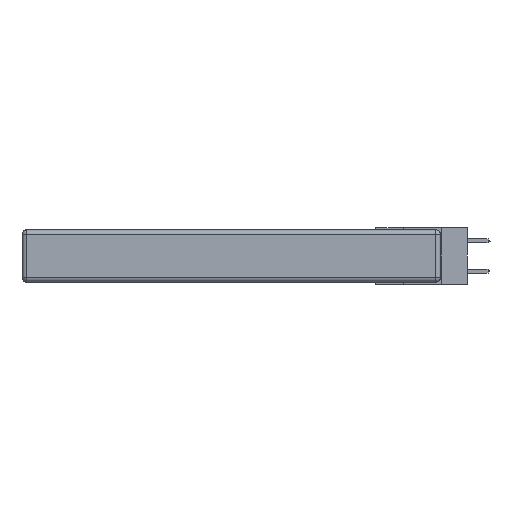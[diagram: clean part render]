
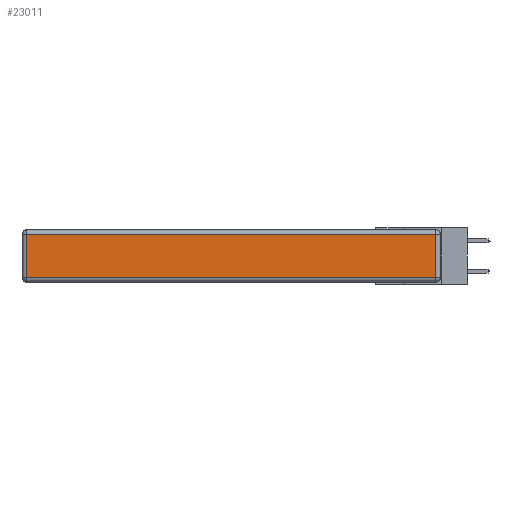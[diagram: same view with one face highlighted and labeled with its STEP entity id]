
A CAD part, left-side view. The second image highlights one B-rep face of the part: STEP entity #23011.
In plain terms, the highlighted planar face has unit normal (-1, 0, 0).
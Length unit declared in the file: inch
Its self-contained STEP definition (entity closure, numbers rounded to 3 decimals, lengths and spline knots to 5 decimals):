
#244 = EDGE_CURVE ( 'NONE', #16506, #13384, #18685, .T. ) ;
#270 = EDGE_CURVE ( 'NONE', #25897, #11508, #22261, .T. ) ;
#1477 = CARTESIAN_POINT ( 'NONE',  ( 0., 2.75, -0.03 ) ) ;
#1549 = ORIENTED_EDGE ( 'NONE', *, *, #270, .T. ) ;
#8575 = DIRECTION ( 'NONE',  ( -1., 0., 0. ) ) ;
#9129 = CARTESIAN_POINT ( 'NONE',  ( 0., 0.03, -0.03 ) ) ;
#9674 = DIRECTION ( 'NONE',  ( 0., 0., -1. ) ) ;
#10591 = VECTOR ( 'NONE', #16017, 39.37008 ) ;
#11338 = DIRECTION ( 'NONE',  ( 0., -1., 0. ) ) ;
#11508 = VERTEX_POINT ( 'NONE', #16377 ) ;
#12030 = ORIENTED_EDGE ( 'NONE', *, *, #14985, .T. ) ;
#13384 = VERTEX_POINT ( 'NONE', #9129 ) ;
#13625 = VECTOR ( 'NONE', #11338, 39.37008 ) ;
#14985 = EDGE_CURVE ( 'NONE', #11508, #16506, #17604, .T. ) ;
#16017 = DIRECTION ( 'NONE',  ( 0., 1., 0. ) ) ;
#16377 = CARTESIAN_POINT ( 'NONE',  ( 0., 2.72, -0.313 ) ) ;
#16506 = VERTEX_POINT ( 'NONE', #28806 ) ;
#16746 = ORIENTED_EDGE ( 'NONE', *, *, #20774, .T. ) ;
#17233 = FACE_OUTER_BOUND ( 'NONE', #24622, .T. ) ;
#17314 = PLANE ( 'NONE',  #20260 ) ;
#17423 = CARTESIAN_POINT ( 'NONE',  ( 0., 0., -0.343 ) ) ;
#17604 = LINE ( 'NONE', #25397, #13625 ) ;
#18685 = LINE ( 'NONE', #23398, #20120 ) ;
#19004 = DIRECTION ( 'NONE',  ( 0., 0., 1. ) ) ;
#19221 = LINE ( 'NONE', #1477, #10591 ) ;
#20120 = VECTOR ( 'NONE', #19004, 39.37008 ) ;
#20260 = AXIS2_PLACEMENT_3D ( 'NONE', #17423, #8575, #24440 ) ;
#20774 = EDGE_CURVE ( 'NONE', #13384, #25897, #19221, .T. ) ;
#20807 = VECTOR ( 'NONE', #9674, 39.37008 ) ;
#21301 = CARTESIAN_POINT ( 'NONE',  ( 0., 2.72, -0.343 ) ) ;
#22261 = LINE ( 'NONE', #21301, #20807 ) ;
#23011 = ADVANCED_FACE ( 'NONE', ( #17233 ), #17314, .T. ) ;
#23104 = ORIENTED_EDGE ( 'NONE', *, *, #244, .T. ) ;
#23285 = CARTESIAN_POINT ( 'NONE',  ( 0., 2.72, -0.03 ) ) ;
#23398 = CARTESIAN_POINT ( 'NONE',  ( 0., 0.03, -0.343 ) ) ;
#24440 = DIRECTION ( 'NONE',  ( 0., 0., 1. ) ) ;
#24622 = EDGE_LOOP ( 'NONE', ( #12030, #23104, #16746, #1549 ) ) ;
#25397 = CARTESIAN_POINT ( 'NONE',  ( 0., 0., -0.313 ) ) ;
#25897 = VERTEX_POINT ( 'NONE', #23285 ) ;
#28806 = CARTESIAN_POINT ( 'NONE',  ( 0., 0.03, -0.313 ) ) ;
